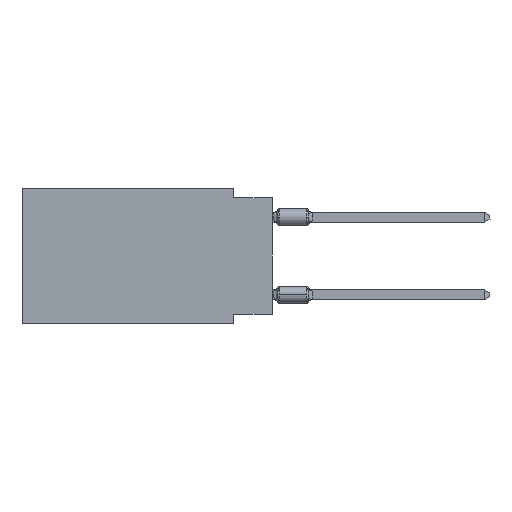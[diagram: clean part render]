
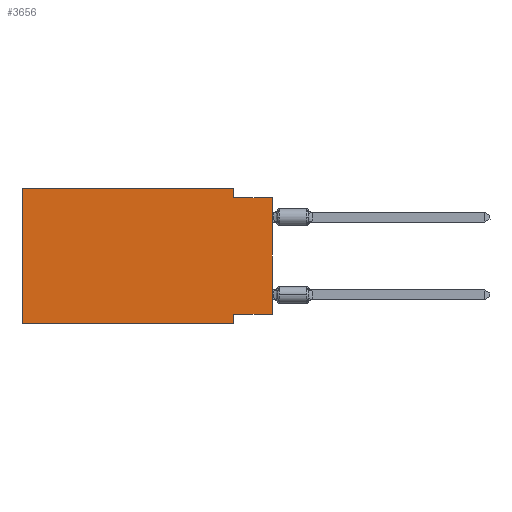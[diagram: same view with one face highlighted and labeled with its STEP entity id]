
A CAD part, left-side view. The second image highlights one B-rep face of the part: STEP entity #3656.
In plain terms, the highlighted planar face has unit normal (-1, 0, 0).
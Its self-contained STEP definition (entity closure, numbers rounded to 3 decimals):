
#578 = VERTEX_POINT ( 'NONE', #16577 ) ;
#950 = EDGE_CURVE ( 'NONE', #23623, #10116, #20104, .T. ) ;
#1642 = LINE ( 'NONE', #3865, #8548 ) ;
#2201 = CARTESIAN_POINT ( 'NONE',  ( 0., 16.383, 0. ) ) ;
#2842 = EDGE_CURVE ( 'NONE', #578, #20418, #1642, .T. ) ;
#3123 = ORIENTED_EDGE ( 'NONE', *, *, #21581, .F. ) ;
#3407 = DIRECTION ( 'NONE',  ( 0., -1., 0. ) ) ;
#3520 = LINE ( 'NONE', #18746, #10799 ) ;
#3656 = ADVANCED_FACE ( 'NONE', ( #15438 ), #5286, .F. ) ;
#3765 = CARTESIAN_POINT ( 'NONE',  ( 0., 0., 0. ) ) ;
#3865 = CARTESIAN_POINT ( 'NONE',  ( 0., 2.54, 0. ) ) ;
#3938 = DIRECTION ( 'NONE',  ( 0., -1., 0. ) ) ;
#5073 = VECTOR ( 'NONE', #21382, 1000. ) ;
#5236 = ORIENTED_EDGE ( 'NONE', *, *, #950, .T. ) ;
#5286 = PLANE ( 'NONE',  #23836 ) ;
#5875 = CARTESIAN_POINT ( 'NONE',  ( 0., 2.54, -0.635 ) ) ;
#6645 = ORIENTED_EDGE ( 'NONE', *, *, #2842, .F. ) ;
#6811 = EDGE_CURVE ( 'NONE', #12516, #22886, #16074, .T. ) ;
#6940 = VECTOR ( 'NONE', #20704, 1000. ) ;
#7071 = EDGE_LOOP ( 'NONE', ( #20162, #14658, #6645, #13937, #10439, #5236, #3123, #20700 ) ) ;
#7338 = DIRECTION ( 'NONE',  ( 0., 0., 1. ) ) ;
#8463 = DIRECTION ( 'NONE',  ( 0., 1., 0. ) ) ;
#8548 = VECTOR ( 'NONE', #18844, 1000. ) ;
#8823 = CARTESIAN_POINT ( 'NONE',  ( 0., 16.383, 0. ) ) ;
#9467 = VERTEX_POINT ( 'NONE', #8823 ) ;
#9715 = CARTESIAN_POINT ( 'NONE',  ( 0., 2.54, -8.89 ) ) ;
#9988 = CARTESIAN_POINT ( 'NONE',  ( 0., 0., -0.635 ) ) ;
#10116 = VERTEX_POINT ( 'NONE', #10589 ) ;
#10381 = CARTESIAN_POINT ( 'NONE',  ( 0., 16.383, -8.89 ) ) ;
#10432 = CARTESIAN_POINT ( 'NONE',  ( 0., 0., -8.255 ) ) ;
#10439 = ORIENTED_EDGE ( 'NONE', *, *, #18710, .F. ) ;
#10589 = CARTESIAN_POINT ( 'NONE',  ( 0., 2.54, -8.89 ) ) ;
#10799 = VECTOR ( 'NONE', #7338, 1000. ) ;
#11675 = DIRECTION ( 'NONE',  ( 0., 0., -1. ) ) ;
#11911 = CARTESIAN_POINT ( 'NONE',  ( 0., 2.54, -8.255 ) ) ;
#12209 = LINE ( 'NONE', #19675, #5073 ) ;
#12515 = CARTESIAN_POINT ( 'NONE',  ( 0., 16.383, -8.89 ) ) ;
#12516 = VERTEX_POINT ( 'NONE', #21422 ) ;
#12527 = VECTOR ( 'NONE', #8463, 1000. ) ;
#13937 = ORIENTED_EDGE ( 'NONE', *, *, #17955, .F. ) ;
#14658 = ORIENTED_EDGE ( 'NONE', *, *, #16447, .F. ) ;
#14961 = LINE ( 'NONE', #3765, #6940 ) ;
#15438 = FACE_OUTER_BOUND ( 'NONE', #7071, .T. ) ;
#15564 = VECTOR ( 'NONE', #11675, 1000. ) ;
#16074 = LINE ( 'NONE', #10432, #12527 ) ;
#16251 = VECTOR ( 'NONE', #3407, 1000. ) ;
#16447 = EDGE_CURVE ( 'NONE', #20418, #16465, #12209, .T. ) ;
#16465 = VERTEX_POINT ( 'NONE', #9988 ) ;
#16577 = CARTESIAN_POINT ( 'NONE',  ( 0., 2.54, 0. ) ) ;
#17048 = VECTOR ( 'NONE', #3938, 1000. ) ;
#17284 = DIRECTION ( 'NONE',  ( 0., 0., -1. ) ) ;
#17955 = EDGE_CURVE ( 'NONE', #9467, #578, #19032, .T. ) ;
#18710 = EDGE_CURVE ( 'NONE', #23623, #9467, #3520, .T. ) ;
#18746 = CARTESIAN_POINT ( 'NONE',  ( 0., 16.383, 0. ) ) ;
#18844 = DIRECTION ( 'NONE',  ( 0., 0., -1. ) ) ;
#19032 = LINE ( 'NONE', #2201, #17048 ) ;
#19675 = CARTESIAN_POINT ( 'NONE',  ( 0., 0., -0.635 ) ) ;
#20104 = LINE ( 'NONE', #12515, #16251 ) ;
#20162 = ORIENTED_EDGE ( 'NONE', *, *, #22106, .T. ) ;
#20418 = VERTEX_POINT ( 'NONE', #5875 ) ;
#20700 = ORIENTED_EDGE ( 'NONE', *, *, #6811, .F. ) ;
#20704 = DIRECTION ( 'NONE',  ( 0., 0., 1. ) ) ;
#20733 = LINE ( 'NONE', #9715, #15564 ) ;
#21382 = DIRECTION ( 'NONE',  ( 0., -1., 0. ) ) ;
#21422 = CARTESIAN_POINT ( 'NONE',  ( 0., 0., -8.255 ) ) ;
#21581 = EDGE_CURVE ( 'NONE', #22886, #10116, #20733, .T. ) ;
#22106 = EDGE_CURVE ( 'NONE', #12516, #16465, #14961, .T. ) ;
#22886 = VERTEX_POINT ( 'NONE', #11911 ) ;
#22921 = CARTESIAN_POINT ( 'NONE',  ( 0., 16.383, 0. ) ) ;
#23623 = VERTEX_POINT ( 'NONE', #10381 ) ;
#23836 = AXIS2_PLACEMENT_3D ( 'NONE', #22921, #24075, #17284 ) ;
#24075 = DIRECTION ( 'NONE',  ( 1., 0., 0. ) ) ;
